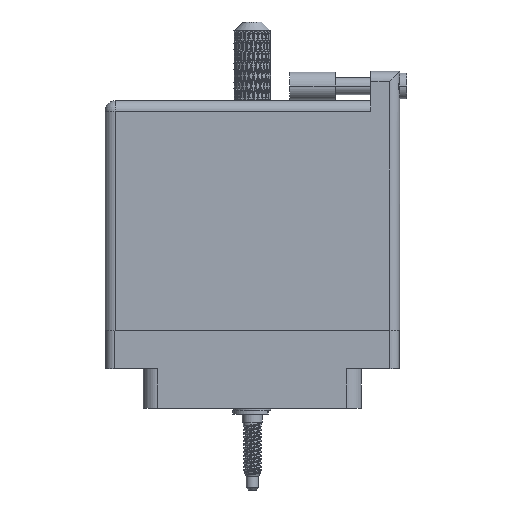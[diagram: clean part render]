
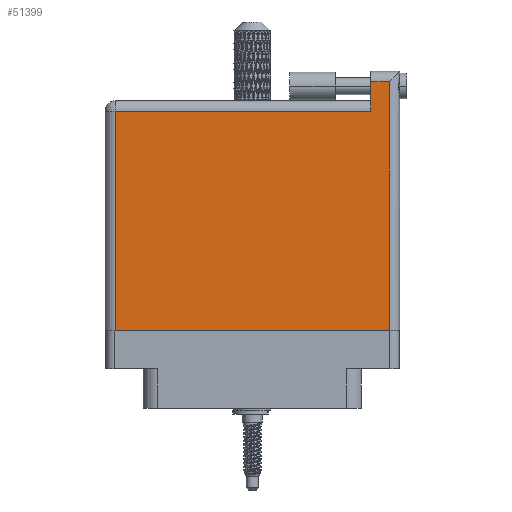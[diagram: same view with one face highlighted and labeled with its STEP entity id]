
A CAD part, front view. The second image highlights one B-rep face of the part: STEP entity #51399.
In plain terms, the highlighted face is planar.
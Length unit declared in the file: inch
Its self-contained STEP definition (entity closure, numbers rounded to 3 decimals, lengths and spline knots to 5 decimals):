
#1281 = EDGE_CURVE ( 'NONE', #66109, #46435, #69499, .T. ) ;
#2459 = LINE ( 'NONE', #35731, #75315 ) ;
#3545 = AXIS2_PLACEMENT_3D ( 'NONE', #71760, #104034, #23649 ) ;
#4486 = DIRECTION ( 'NONE',  ( -1., 0., 0. ) ) ;
#6555 = CARTESIAN_POINT ( 'NONE',  ( 1.938, 1.696, 0. ) ) ;
#10863 = ORIENTED_EDGE ( 'NONE', *, *, #22602, .T. ) ;
#14310 = CARTESIAN_POINT ( 'NONE',  ( 0., 1.496, 0. ) ) ;
#17751 = VECTOR ( 'NONE', #46558, 39.37008 ) ;
#18056 = ORIENTED_EDGE ( 'NONE', *, *, #50445, .T. ) ;
#21478 = VERTEX_POINT ( 'NONE', #65432 ) ;
#22602 = EDGE_CURVE ( 'NONE', #60825, #83201, #2459, .T. ) ;
#23649 = DIRECTION ( 'NONE',  ( -1., 0., 0. ) ) ;
#25628 = LINE ( 'NONE', #88586, #62474 ) ;
#26267 = CARTESIAN_POINT ( 'NONE',  ( 1.938, 1.766, 0. ) ) ;
#26524 = ORIENTED_EDGE ( 'NONE', *, *, #98670, .T. ) ;
#27369 = CARTESIAN_POINT ( 'NONE',  ( 0., 0., 0. ) ) ;
#28174 = ORIENTED_EDGE ( 'NONE', *, *, #70110, .T. ) ;
#31240 = CARTESIAN_POINT ( 'NONE',  ( 1.811, 1.696, 0. ) ) ;
#34690 = DIRECTION ( 'NONE',  ( 0., -1., 0. ) ) ;
#35253 = CARTESIAN_POINT ( 'NONE',  ( 1.938, 0., 0. ) ) ;
#35731 = CARTESIAN_POINT ( 'NONE',  ( 0.07, 0., 0. ) ) ;
#39002 = PLANE ( 'NONE',  #3545 ) ;
#39301 = VERTEX_POINT ( 'NONE', #35253 ) ;
#39532 = VECTOR ( 'NONE', #90789, 39.37008 ) ;
#46435 = VERTEX_POINT ( 'NONE', #31240 ) ;
#46554 = ORIENTED_EDGE ( 'NONE', *, *, #47082, .T. ) ;
#46558 = DIRECTION ( 'NONE',  ( -1., 0., 0. ) ) ;
#47082 = EDGE_CURVE ( 'NONE', #46435, #21478, #25628, .T. ) ;
#50445 = EDGE_CURVE ( 'NONE', #83201, #39301, #51716, .T. ) ;
#51399 = ADVANCED_FACE ( 'NONE', ( #102999 ), #39002, .F. ) ;
#51716 = LINE ( 'NONE', #27369, #79003 ) ;
#52389 = ORIENTED_EDGE ( 'NONE', *, *, #1281, .T. ) ;
#54188 = CARTESIAN_POINT ( 'NONE',  ( 0., 1.696, 0. ) ) ;
#57884 = DIRECTION ( 'NONE',  ( 0., -1., 0. ) ) ;
#59635 = DIRECTION ( 'NONE',  ( 1., 0., 0. ) ) ;
#60825 = VERTEX_POINT ( 'NONE', #66305 ) ;
#62474 = VECTOR ( 'NONE', #57884, 39.37008 ) ;
#65432 = CARTESIAN_POINT ( 'NONE',  ( 1.811, 1.496, 0. ) ) ;
#66109 = VERTEX_POINT ( 'NONE', #6555 ) ;
#66305 = CARTESIAN_POINT ( 'NONE',  ( 0.07, 1.496, 0. ) ) ;
#69276 = LINE ( 'NONE', #14310, #17751 ) ;
#69499 = LINE ( 'NONE', #54188, #82050 ) ;
#70110 = EDGE_CURVE ( 'NONE', #21478, #60825, #69276, .T. ) ;
#71760 = CARTESIAN_POINT ( 'NONE',  ( 0., 1.566, 0. ) ) ;
#75259 = CARTESIAN_POINT ( 'NONE',  ( 0.07, 0., 0. ) ) ;
#75315 = VECTOR ( 'NONE', #34690, 39.37008 ) ;
#79003 = VECTOR ( 'NONE', #59635, 39.37008 ) ;
#79870 = LINE ( 'NONE', #26267, #39532 ) ;
#82050 = VECTOR ( 'NONE', #4486, 39.37008 ) ;
#83201 = VERTEX_POINT ( 'NONE', #75259 ) ;
#88586 = CARTESIAN_POINT ( 'NONE',  ( 1.811, 1.766, 0. ) ) ;
#90789 = DIRECTION ( 'NONE',  ( 0., 1., 0. ) ) ;
#92278 = EDGE_LOOP ( 'NONE', ( #18056, #26524, #52389, #46554, #28174, #10863 ) ) ;
#98670 = EDGE_CURVE ( 'NONE', #39301, #66109, #79870, .T. ) ;
#102999 = FACE_OUTER_BOUND ( 'NONE', #92278, .T. ) ;
#104034 = DIRECTION ( 'NONE',  ( 0., 0., -1. ) ) ;
